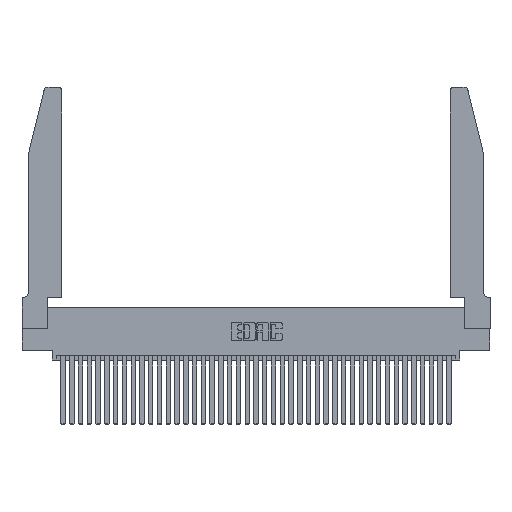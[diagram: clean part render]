
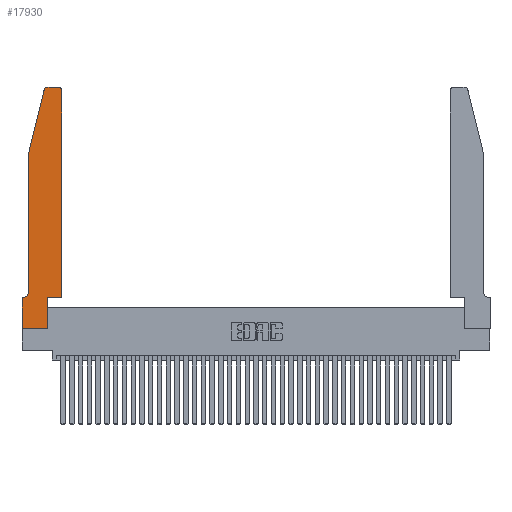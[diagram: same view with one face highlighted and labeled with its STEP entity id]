
A CAD part, top view. The second image highlights one B-rep face of the part: STEP entity #17930.
In plain terms, the highlighted planar face has unit normal (0, 0, 1).
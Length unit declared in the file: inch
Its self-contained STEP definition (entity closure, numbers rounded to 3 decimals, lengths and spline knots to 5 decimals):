
#289 = LINE ( 'NONE', #19094, #31942 ) ;
#1463 = ORIENTED_EDGE ( 'NONE', *, *, #25707, .T. ) ;
#1544 = DIRECTION ( 'NONE',  ( 0., 0., 1. ) ) ;
#1643 = VERTEX_POINT ( 'NONE', #12144 ) ;
#2785 = CARTESIAN_POINT ( 'NONE',  ( 0.0755, 2., 0.37 ) ) ;
#3150 = ORIENTED_EDGE ( 'NONE', *, *, #20819, .T. ) ;
#3391 = VECTOR ( 'NONE', #16001, 39.37008 ) ;
#3786 = CARTESIAN_POINT ( 'NONE',  ( 0.284, 2.72, 0.37 ) ) ;
#4788 = EDGE_CURVE ( 'NONE', #5856, #19422, #29316, .T. ) ;
#5459 = CARTESIAN_POINT ( 'NONE',  ( 0., 0.35, 0.37 ) ) ;
#5710 = LINE ( 'NONE', #23656, #29154 ) ;
#5856 = VERTEX_POINT ( 'NONE', #38410 ) ;
#6119 = VERTEX_POINT ( 'NONE', #6292 ) ;
#6292 = CARTESIAN_POINT ( 'NONE',  ( 0.2865, 0.35, 0.37 ) ) ;
#6577 = CARTESIAN_POINT ( 'NONE',  ( 0.0055, 0.35, 0.37 ) ) ;
#6927 = DIRECTION ( 'NONE',  ( 1., 0., 0. ) ) ;
#7790 = CARTESIAN_POINT ( 'NONE',  ( 0.0055, 0.42, 0.37 ) ) ;
#7974 = DIRECTION ( 'NONE',  ( 0., 1., 0. ) ) ;
#8055 = ORIENTED_EDGE ( 'NONE', *, *, #4788, .T. ) ;
#8232 = LINE ( 'NONE', #26265, #24504 ) ;
#8488 = LINE ( 'NONE', #39150, #37069 ) ;
#8635 = VECTOR ( 'NONE', #20514, 39.37008 ) ;
#8661 = DIRECTION ( 'NONE',  ( -1., 0., 0. ) ) ;
#8771 = CARTESIAN_POINT ( 'NONE',  ( 0.0755, 2., 0.37 ) ) ;
#9902 = CARTESIAN_POINT ( 'NONE',  ( 0.2865, 0., 0.37 ) ) ;
#10707 = VERTEX_POINT ( 'NONE', #8771 ) ;
#10883 = DIRECTION ( 'NONE',  ( -1., 0., 0. ) ) ;
#11544 = ORIENTED_EDGE ( 'NONE', *, *, #21635, .T. ) ;
#11704 = CARTESIAN_POINT ( 'NONE',  ( 0.4505, 2.72, 0.37 ) ) ;
#11777 = CARTESIAN_POINT ( 'NONE',  ( 0.2605, 2.75, 0.37 ) ) ;
#11824 = CARTESIAN_POINT ( 'NONE',  ( 0.4505, 0.35, 0.37 ) ) ;
#12144 = CARTESIAN_POINT ( 'NONE',  ( 0., 0., 0.37 ) ) ;
#12473 = ORIENTED_EDGE ( 'NONE', *, *, #38830, .T. ) ;
#14032 = ORIENTED_EDGE ( 'NONE', *, *, #25628, .T. ) ;
#14242 = ORIENTED_EDGE ( 'NONE', *, *, #15879, .T. ) ;
#14254 = CARTESIAN_POINT ( 'NONE',  ( 0.0755, 0.42, 0.37 ) ) ;
#14818 = DIRECTION ( 'NONE',  ( 1., 0., 0. ) ) ;
#14967 = CARTESIAN_POINT ( 'NONE',  ( 0., 0.35, 0.37 ) ) ;
#15719 = CARTESIAN_POINT ( 'NONE',  ( 0.284, 2.75, 0.37 ) ) ;
#15858 = EDGE_CURVE ( 'NONE', #10707, #29615, #18762, .T. ) ;
#15879 = EDGE_CURVE ( 'NONE', #19422, #36305, #26888, .T. ) ;
#16001 = DIRECTION ( 'NONE',  ( 0., -1., 0. ) ) ;
#16750 = LINE ( 'NONE', #32614, #8635 ) ;
#17323 = LINE ( 'NONE', #31782, #32543 ) ;
#17446 = VERTEX_POINT ( 'NONE', #6577 ) ;
#17930 = ADVANCED_FACE ( 'NONE', ( #20974 ), #33196, .T. ) ;
#18039 = DIRECTION ( 'NONE',  ( 0., 0., 1. ) ) ;
#18359 = CARTESIAN_POINT ( 'NONE',  ( 0.25487, 2.72718, 0.37 ) ) ;
#18762 = LINE ( 'NONE', #34218, #3391 ) ;
#19094 = CARTESIAN_POINT ( 'NONE',  ( 0., 0., 0.37 ) ) ;
#19162 = ORIENTED_EDGE ( 'NONE', *, *, #20471, .T. ) ;
#19422 = VERTEX_POINT ( 'NONE', #15719 ) ;
#19944 = CARTESIAN_POINT ( 'NONE',  ( 0.4205, 2.72, 0.37 ) ) ;
#20471 = EDGE_CURVE ( 'NONE', #37674, #30209, #5710, .T. ) ;
#20483 = ORIENTED_EDGE ( 'NONE', *, *, #34967, .T. ) ;
#20487 = VERTEX_POINT ( 'NONE', #5459 ) ;
#20514 = DIRECTION ( 'NONE',  ( -1., 0., 0. ) ) ;
#20713 = VECTOR ( 'NONE', #24120, 39.37008 ) ;
#20769 = VERTEX_POINT ( 'NONE', #9902 ) ;
#20819 = EDGE_CURVE ( 'NONE', #1643, #20769, #289, .T. ) ;
#20974 = FACE_OUTER_BOUND ( 'NONE', #31217, .T. ) ;
#20992 = CIRCLE ( 'NONE', #35222, 0.03 ) ;
#21185 = VECTOR ( 'NONE', #8661, 39.37008 ) ;
#21213 = ORIENTED_EDGE ( 'NONE', *, *, #15858, .T. ) ;
#21635 = EDGE_CURVE ( 'NONE', #30209, #5856, #20992, .T. ) ;
#21672 = LINE ( 'NONE', #2785, #20713 ) ;
#23033 = DIRECTION ( 'NONE',  ( 1., 0., 0. ) ) ;
#23093 = ORIENTED_EDGE ( 'NONE', *, *, #33336, .T. ) ;
#23534 = CIRCLE ( 'NONE', #33483, 0.07 ) ;
#23656 = CARTESIAN_POINT ( 'NONE',  ( 0.4505, 0.35, 0.37 ) ) ;
#24120 = DIRECTION ( 'NONE',  ( -0.239, -0.971, 0. ) ) ;
#24356 = ORIENTED_EDGE ( 'NONE', *, *, #27241, .T. ) ;
#24504 = VECTOR ( 'NONE', #7974, 39.37008 ) ;
#25223 = DIRECTION ( 'NONE',  ( 0., 0., 1. ) ) ;
#25628 = EDGE_CURVE ( 'NONE', #20487, #1643, #17323, .T. ) ;
#25703 = DIRECTION ( 'NONE',  ( 0., -1., 0. ) ) ;
#25707 = EDGE_CURVE ( 'NONE', #29615, #17446, #23534, .T. ) ;
#26265 = CARTESIAN_POINT ( 'NONE',  ( 0.2865, 0.35, 0.37 ) ) ;
#26736 = DIRECTION ( 'NONE',  ( 0., 1., 0. ) ) ;
#26888 = CIRCLE ( 'NONE', #29038, 0.03 ) ;
#27241 = EDGE_CURVE ( 'NONE', #36305, #10707, #21672, .T. ) ;
#28570 = AXIS2_PLACEMENT_3D ( 'NONE', #14967, #18039, #39311 ) ;
#29038 = AXIS2_PLACEMENT_3D ( 'NONE', #3786, #25223, #6927 ) ;
#29152 = DIRECTION ( 'NONE',  ( 0., 0., -1. ) ) ;
#29154 = VECTOR ( 'NONE', #26736, 39.37008 ) ;
#29316 = LINE ( 'NONE', #11777, #21185 ) ;
#29615 = VERTEX_POINT ( 'NONE', #14254 ) ;
#30209 = VERTEX_POINT ( 'NONE', #11704 ) ;
#31217 = EDGE_LOOP ( 'NONE', ( #8055, #14242, #24356, #21213, #1463, #23093, #14032, #3150, #12473, #20483, #19162, #11544 ) ) ;
#31336 = DIRECTION ( 'NONE',  ( 1., 0., 0. ) ) ;
#31782 = CARTESIAN_POINT ( 'NONE',  ( 0., 0., 0.37 ) ) ;
#31942 = VECTOR ( 'NONE', #31336, 39.37008 ) ;
#32543 = VECTOR ( 'NONE', #25703, 39.37008 ) ;
#32614 = CARTESIAN_POINT ( 'NONE',  ( 0.0755, 0.35, 0.37 ) ) ;
#33196 = PLANE ( 'NONE',  #28570 ) ;
#33336 = EDGE_CURVE ( 'NONE', #17446, #20487, #16750, .T. ) ;
#33483 = AXIS2_PLACEMENT_3D ( 'NONE', #7790, #29152, #10883 ) ;
#34218 = CARTESIAN_POINT ( 'NONE',  ( 0.0755, 2., 0.37 ) ) ;
#34967 = EDGE_CURVE ( 'NONE', #6119, #37674, #8488, .T. ) ;
#35222 = AXIS2_PLACEMENT_3D ( 'NONE', #19944, #1544, #23033 ) ;
#36305 = VERTEX_POINT ( 'NONE', #18359 ) ;
#37069 = VECTOR ( 'NONE', #14818, 39.37008 ) ;
#37674 = VERTEX_POINT ( 'NONE', #11824 ) ;
#38410 = CARTESIAN_POINT ( 'NONE',  ( 0.4205, 2.75, 0.37 ) ) ;
#38830 = EDGE_CURVE ( 'NONE', #20769, #6119, #8232, .T. ) ;
#39150 = CARTESIAN_POINT ( 'NONE',  ( 0.4505, 0.35, 0.37 ) ) ;
#39311 = DIRECTION ( 'NONE',  ( 1., 0., 0. ) ) ;
